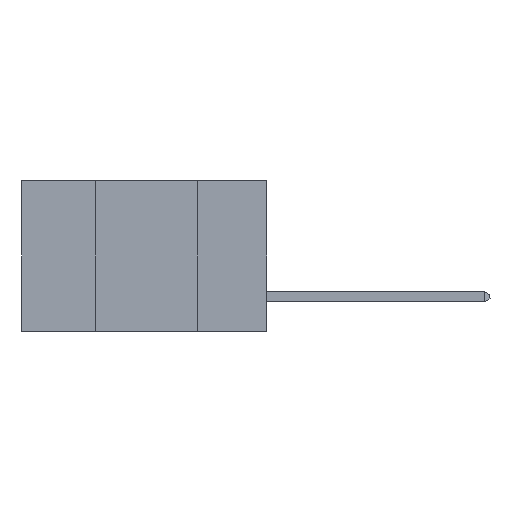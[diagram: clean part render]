
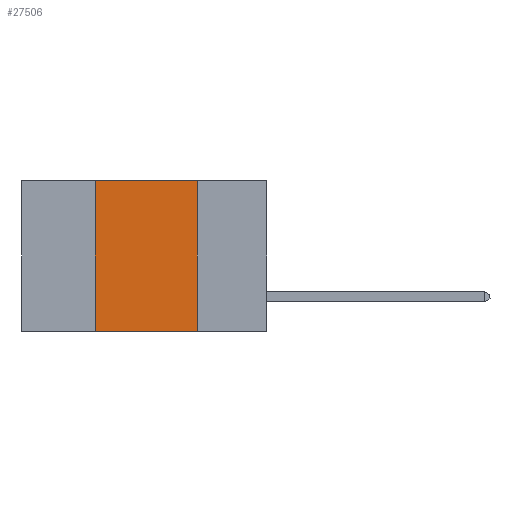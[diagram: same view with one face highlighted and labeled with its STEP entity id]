
A CAD part, left-side view. The second image highlights one B-rep face of the part: STEP entity #27506.
In plain terms, the highlighted planar face has unit normal (-1, 0, 0).
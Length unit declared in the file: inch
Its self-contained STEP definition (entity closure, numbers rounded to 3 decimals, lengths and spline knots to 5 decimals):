
#365 = VECTOR ( 'NONE', #1771, 39.37008 ) ;
#1771 = DIRECTION ( 'NONE',  ( 0., 0., 1. ) ) ;
#2863 = VERTEX_POINT ( 'NONE', #13722 ) ;
#4871 = CARTESIAN_POINT ( 'NONE',  ( 0., 0.6, 0. ) ) ;
#6871 = VECTOR ( 'NONE', #32103, 39.37008 ) ;
#7326 = DIRECTION ( 'NONE',  ( 0., 0., -1. ) ) ;
#7721 = EDGE_LOOP ( 'NONE', ( #27419, #23578, #32465, #29022 ) ) ;
#7912 = DIRECTION ( 'NONE',  ( 0., 0., -1. ) ) ;
#10866 = VECTOR ( 'NONE', #31652, 39.37008 ) ;
#11318 = CARTESIAN_POINT ( 'NONE',  ( 0., 0.42, -0.37 ) ) ;
#12170 = FACE_OUTER_BOUND ( 'NONE', #7721, .T. ) ;
#13722 = CARTESIAN_POINT ( 'NONE',  ( 0., 0.17, 0. ) ) ;
#14124 = CARTESIAN_POINT ( 'NONE',  ( 0., 0.17, -0.37 ) ) ;
#15694 = EDGE_CURVE ( 'NONE', #30490, #2863, #19910, .T. ) ;
#16557 = LINE ( 'NONE', #16921, #365 ) ;
#16921 = CARTESIAN_POINT ( 'NONE',  ( 0., 0.42, 0. ) ) ;
#18454 = VERTEX_POINT ( 'NONE', #11318 ) ;
#18692 = VECTOR ( 'NONE', #7326, 39.37008 ) ;
#19652 = AXIS2_PLACEMENT_3D ( 'NONE', #4871, #26172, #7912 ) ;
#19910 = LINE ( 'NONE', #37495, #10866 ) ;
#23578 = ORIENTED_EDGE ( 'NONE', *, *, #15694, .F. ) ;
#26172 = DIRECTION ( 'NONE',  ( 1., 0., 0. ) ) ;
#27419 = ORIENTED_EDGE ( 'NONE', *, *, #34266, .F. ) ;
#27506 = ADVANCED_FACE ( 'NONE', ( #12170 ), #38000, .F. ) ;
#28599 = CARTESIAN_POINT ( 'NONE',  ( 0., 0.17, 0. ) ) ;
#29022 = ORIENTED_EDGE ( 'NONE', *, *, #32494, .T. ) ;
#29106 = CARTESIAN_POINT ( 'NONE',  ( 0., 0.6, -0.37 ) ) ;
#30490 = VERTEX_POINT ( 'NONE', #32663 ) ;
#30993 = EDGE_CURVE ( 'NONE', #18454, #30490, #16557, .T. ) ;
#31089 = LINE ( 'NONE', #29106, #6871 ) ;
#31652 = DIRECTION ( 'NONE',  ( 0., -1., 0. ) ) ;
#32103 = DIRECTION ( 'NONE',  ( 0., -1., 0. ) ) ;
#32465 = ORIENTED_EDGE ( 'NONE', *, *, #30993, .F. ) ;
#32494 = EDGE_CURVE ( 'NONE', #18454, #37424, #31089, .T. ) ;
#32663 = CARTESIAN_POINT ( 'NONE',  ( 0., 0.42, 0. ) ) ;
#34266 = EDGE_CURVE ( 'NONE', #2863, #37424, #35654, .T. ) ;
#35654 = LINE ( 'NONE', #28599, #18692 ) ;
#37424 = VERTEX_POINT ( 'NONE', #14124 ) ;
#37495 = CARTESIAN_POINT ( 'NONE',  ( 0., 0.6, 0. ) ) ;
#38000 = PLANE ( 'NONE',  #19652 ) ;
